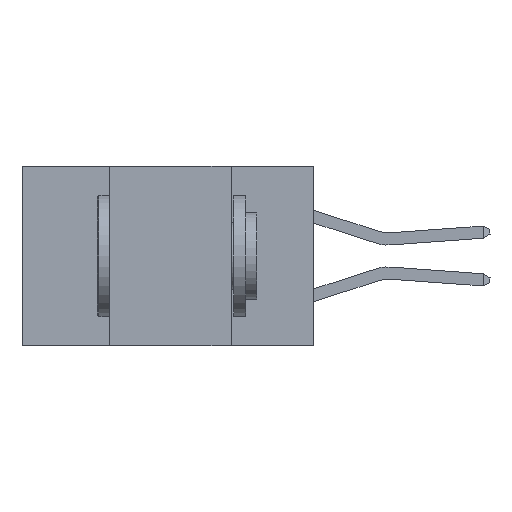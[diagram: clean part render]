
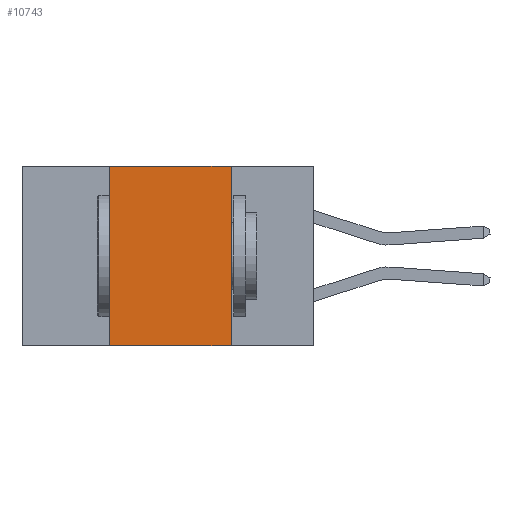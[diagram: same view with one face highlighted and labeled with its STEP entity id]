
A CAD part, left-side view. The second image highlights one B-rep face of the part: STEP entity #10743.
In plain terms, the highlighted planar face has unit normal (-1, 0, 0).
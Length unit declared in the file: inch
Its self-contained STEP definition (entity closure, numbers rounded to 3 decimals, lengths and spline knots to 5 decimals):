
#114 = CARTESIAN_POINT ( 'NONE',  ( 0., 0.42, 0. ) ) ;
#140 = VECTOR ( 'NONE', #2480, 39.37008 ) ;
#704 = DIRECTION ( 'NONE',  ( 0., 0., -1. ) ) ;
#711 = CARTESIAN_POINT ( 'NONE',  ( 0., 0.17, -0.37 ) ) ;
#1268 = FACE_OUTER_BOUND ( 'NONE', #1893, .T. ) ;
#1544 = VECTOR ( 'NONE', #8519, 39.37008 ) ;
#1893 = EDGE_LOOP ( 'NONE', ( #6164, #3593, #11009, #9648 ) ) ;
#2480 = DIRECTION ( 'NONE',  ( 0., -1., 0. ) ) ;
#2651 = LINE ( 'NONE', #10283, #140 ) ;
#3309 = VERTEX_POINT ( 'NONE', #6094 ) ;
#3593 = ORIENTED_EDGE ( 'NONE', *, *, #11196, .F. ) ;
#3927 = VERTEX_POINT ( 'NONE', #5559 ) ;
#4215 = DIRECTION ( 'NONE',  ( 0., 0., -1. ) ) ;
#4373 = LINE ( 'NONE', #6025, #5870 ) ;
#4652 = EDGE_CURVE ( 'NONE', #3309, #8930, #4373, .T. ) ;
#5227 = DIRECTION ( 'NONE',  ( 0., -1., 0. ) ) ;
#5559 = CARTESIAN_POINT ( 'NONE',  ( 0., 0.42, -0.37 ) ) ;
#5870 = VECTOR ( 'NONE', #4215, 39.37008 ) ;
#6025 = CARTESIAN_POINT ( 'NONE',  ( 0., 0.17, 0. ) ) ;
#6094 = CARTESIAN_POINT ( 'NONE',  ( 0., 0.17, 0. ) ) ;
#6164 = ORIENTED_EDGE ( 'NONE', *, *, #4652, .F. ) ;
#6345 = LINE ( 'NONE', #7089, #7655 ) ;
#7089 = CARTESIAN_POINT ( 'NONE',  ( 0., 0.6, 0. ) ) ;
#7411 = CARTESIAN_POINT ( 'NONE',  ( 0., 0.42, 0. ) ) ;
#7511 = LINE ( 'NONE', #114, #1544 ) ;
#7655 = VECTOR ( 'NONE', #5227, 39.37008 ) ;
#8273 = EDGE_CURVE ( 'NONE', #3927, #8930, #2651, .T. ) ;
#8371 = DIRECTION ( 'NONE',  ( 1., 0., 0. ) ) ;
#8519 = DIRECTION ( 'NONE',  ( 0., 0., 1. ) ) ;
#8930 = VERTEX_POINT ( 'NONE', #711 ) ;
#9298 = CARTESIAN_POINT ( 'NONE',  ( 0., 0.6, 0. ) ) ;
#9648 = ORIENTED_EDGE ( 'NONE', *, *, #8273, .T. ) ;
#10283 = CARTESIAN_POINT ( 'NONE',  ( 0., 0.6, -0.37 ) ) ;
#10302 = AXIS2_PLACEMENT_3D ( 'NONE', #9298, #8371, #704 ) ;
#10456 = VERTEX_POINT ( 'NONE', #7411 ) ;
#10743 = ADVANCED_FACE ( 'NONE', ( #1268 ), #12338, .F. ) ;
#11009 = ORIENTED_EDGE ( 'NONE', *, *, #11130, .F. ) ;
#11130 = EDGE_CURVE ( 'NONE', #3927, #10456, #7511, .T. ) ;
#11196 = EDGE_CURVE ( 'NONE', #10456, #3309, #6345, .T. ) ;
#12338 = PLANE ( 'NONE',  #10302 ) ;
